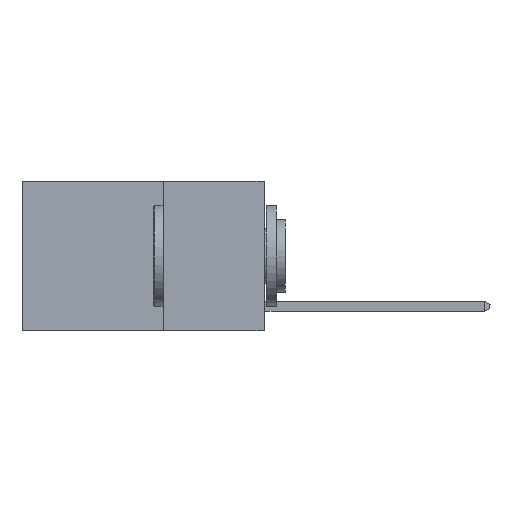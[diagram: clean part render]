
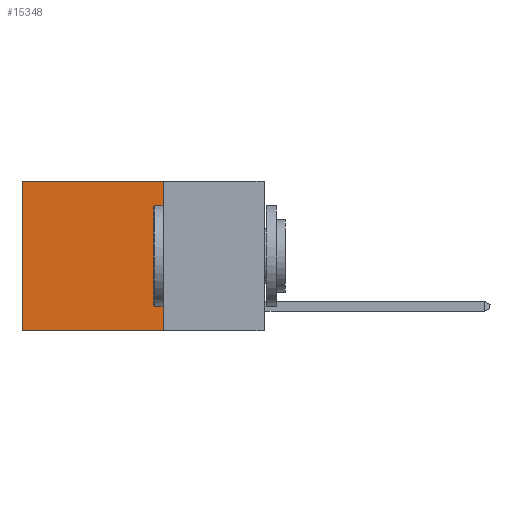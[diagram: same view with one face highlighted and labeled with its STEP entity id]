
A CAD part, left-side view. The second image highlights one B-rep face of the part: STEP entity #15348.
In plain terms, the highlighted planar face has unit normal (-1, 0, 0).
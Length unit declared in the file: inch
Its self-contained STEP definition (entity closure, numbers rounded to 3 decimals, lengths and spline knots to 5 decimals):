
#669 = LINE ( 'NONE', #6581, #19486 ) ;
#1183 = EDGE_CURVE ( 'NONE', #1407, #22745, #669, .T. ) ;
#1378 = CARTESIAN_POINT ( 'NONE',  ( 0.2625, 0.25, 0. ) ) ;
#1407 = VERTEX_POINT ( 'NONE', #5498 ) ;
#1764 = CARTESIAN_POINT ( 'NONE',  ( 0.2625, 0.6, -0.37 ) ) ;
#1843 = AXIS2_PLACEMENT_3D ( 'NONE', #1378, #17339, #6732 ) ;
#1884 = VECTOR ( 'NONE', #22730, 39.37008 ) ;
#2179 = DIRECTION ( 'NONE',  ( 0., 1., 0. ) ) ;
#3010 = FACE_OUTER_BOUND ( 'NONE', #4136, .T. ) ;
#3572 = CARTESIAN_POINT ( 'NONE',  ( 0.2625, 0.25, -0.37 ) ) ;
#4136 = EDGE_LOOP ( 'NONE', ( #9143, #12452, #9483, #16460 ) ) ;
#4646 = VECTOR ( 'NONE', #20087, 39.37008 ) ;
#5498 = CARTESIAN_POINT ( 'NONE',  ( 0.2625, 0.6, 0. ) ) ;
#6581 = CARTESIAN_POINT ( 'NONE',  ( 0.2625, 0.6, 0. ) ) ;
#6732 = DIRECTION ( 'NONE',  ( 0., 0., -1. ) ) ;
#7380 = EDGE_CURVE ( 'NONE', #14585, #22745, #13829, .T. ) ;
#7626 = CARTESIAN_POINT ( 'NONE',  ( 0.2625, 0.25, 0. ) ) ;
#9143 = ORIENTED_EDGE ( 'NONE', *, *, #1183, .T. ) ;
#9378 = LINE ( 'NONE', #9437, #4646 ) ;
#9437 = CARTESIAN_POINT ( 'NONE',  ( 0.2625, 0.25, 0. ) ) ;
#9483 = ORIENTED_EDGE ( 'NONE', *, *, #15684, .F. ) ;
#12452 = ORIENTED_EDGE ( 'NONE', *, *, #7380, .F. ) ;
#13829 = LINE ( 'NONE', #16349, #18554 ) ;
#14585 = VERTEX_POINT ( 'NONE', #3572 ) ;
#15348 = ADVANCED_FACE ( 'NONE', ( #3010 ), #15554, .F. ) ;
#15419 = EDGE_CURVE ( 'NONE', #16831, #1407, #16017, .T. ) ;
#15554 = PLANE ( 'NONE',  #1843 ) ;
#15684 = EDGE_CURVE ( 'NONE', #16831, #14585, #9378, .T. ) ;
#15708 = CARTESIAN_POINT ( 'NONE',  ( 0.2625, 0.25, 0. ) ) ;
#16017 = LINE ( 'NONE', #15708, #1884 ) ;
#16349 = CARTESIAN_POINT ( 'NONE',  ( 0.2625, 0.25, -0.37 ) ) ;
#16460 = ORIENTED_EDGE ( 'NONE', *, *, #15419, .T. ) ;
#16831 = VERTEX_POINT ( 'NONE', #7626 ) ;
#17197 = DIRECTION ( 'NONE',  ( 0., 0., -1. ) ) ;
#17339 = DIRECTION ( 'NONE',  ( 1., 0., 0. ) ) ;
#18554 = VECTOR ( 'NONE', #2179, 39.37008 ) ;
#19486 = VECTOR ( 'NONE', #17197, 39.37008 ) ;
#20087 = DIRECTION ( 'NONE',  ( 0., 0., -1. ) ) ;
#22730 = DIRECTION ( 'NONE',  ( 0., 1., 0. ) ) ;
#22745 = VERTEX_POINT ( 'NONE', #1764 ) ;
